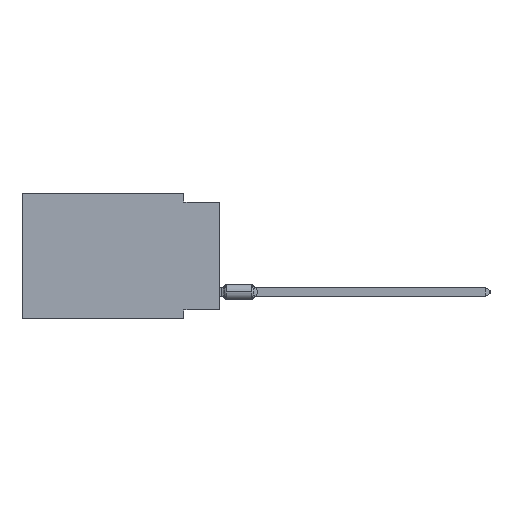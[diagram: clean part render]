
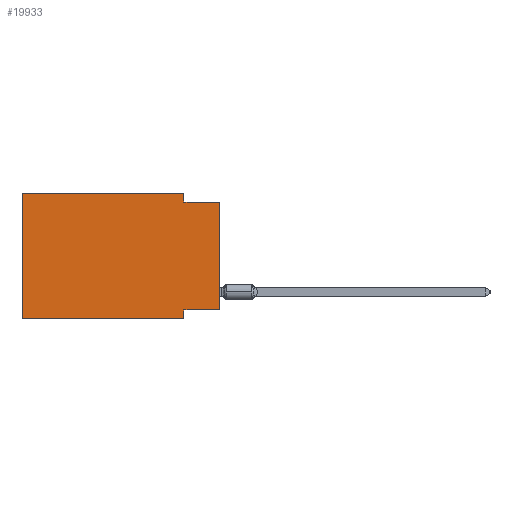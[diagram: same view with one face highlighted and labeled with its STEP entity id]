
A CAD part, left-side view. The second image highlights one B-rep face of the part: STEP entity #19933.
In plain terms, the highlighted planar face has unit normal (-1, 0, 0).
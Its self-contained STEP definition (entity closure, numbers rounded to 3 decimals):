
#3803 = DIRECTION ( 'NONE',  ( 0., 0., 1. ) ) ;
#4120 = EDGE_CURVE ( 'NONE', #29548, #60700, #34407, .T. ) ;
#5453 = VERTEX_POINT ( 'NONE', #26702 ) ;
#8085 = LINE ( 'NONE', #81244, #57320 ) ;
#9724 = CARTESIAN_POINT ( 'NONE',  ( 0., 2.54, 0. ) ) ;
#10638 = CARTESIAN_POINT ( 'NONE',  ( 0., 13.97, 0. ) ) ;
#11096 = CARTESIAN_POINT ( 'NONE',  ( 0., 2.54, -8.89 ) ) ;
#13629 = DIRECTION ( 'NONE',  ( 0., 1., 0. ) ) ;
#16205 = ORIENTED_EDGE ( 'NONE', *, *, #82289, .F. ) ;
#17096 = PLANE ( 'NONE',  #102132 ) ;
#19933 = ADVANCED_FACE ( 'NONE', ( #73169 ), #17096, .F. ) ;
#20135 = DIRECTION ( 'NONE',  ( 0., 0., -1. ) ) ;
#25701 = DIRECTION ( 'NONE',  ( 0., -1., 0. ) ) ;
#26398 = DIRECTION ( 'NONE',  ( 0., -1., 0. ) ) ;
#26702 = CARTESIAN_POINT ( 'NONE',  ( 0., 0., -8.255 ) ) ;
#27596 = VECTOR ( 'NONE', #26398, 1000. ) ;
#27738 = CARTESIAN_POINT ( 'NONE',  ( 0., 0., -0.635 ) ) ;
#28299 = ORIENTED_EDGE ( 'NONE', *, *, #104268, .T. ) ;
#28945 = EDGE_CURVE ( 'NONE', #60700, #82706, #66295, .T. ) ;
#29548 = VERTEX_POINT ( 'NONE', #10638 ) ;
#31070 = ORIENTED_EDGE ( 'NONE', *, *, #4120, .F. ) ;
#31104 = DIRECTION ( 'NONE',  ( 0., 0., 1. ) ) ;
#32250 = EDGE_CURVE ( 'NONE', #67128, #29548, #66833, .T. ) ;
#33915 = ORIENTED_EDGE ( 'NONE', *, *, #34545, .F. ) ;
#34407 = LINE ( 'NONE', #66945, #27596 ) ;
#34545 = EDGE_CURVE ( 'NONE', #82706, #63183, #56461, .T. ) ;
#39136 = LINE ( 'NONE', #72200, #97717 ) ;
#41253 = DIRECTION ( 'NONE',  ( 0., 0., -1. ) ) ;
#43645 = DIRECTION ( 'NONE',  ( 0., 0., -1. ) ) ;
#44591 = CARTESIAN_POINT ( 'NONE',  ( 0., 2.54, 0. ) ) ;
#45098 = CARTESIAN_POINT ( 'NONE',  ( 0., 2.54, -8.89 ) ) ;
#46465 = EDGE_CURVE ( 'NONE', #5453, #63183, #39136, .T. ) ;
#47699 = ORIENTED_EDGE ( 'NONE', *, *, #32250, .F. ) ;
#48477 = DIRECTION ( 'NONE',  ( 0., -1., 0. ) ) ;
#50919 = VECTOR ( 'NONE', #13629, 1000. ) ;
#54197 = CARTESIAN_POINT ( 'NONE',  ( 0., 0., -8.255 ) ) ;
#56028 = VECTOR ( 'NONE', #3803, 1000. ) ;
#56461 = LINE ( 'NONE', #89075, #79188 ) ;
#57320 = VECTOR ( 'NONE', #25701, 1000. ) ;
#59254 = CARTESIAN_POINT ( 'NONE',  ( 0., 2.54, -8.255 ) ) ;
#60700 = VERTEX_POINT ( 'NONE', #44591 ) ;
#61387 = ORIENTED_EDGE ( 'NONE', *, *, #85393, .F. ) ;
#63183 = VERTEX_POINT ( 'NONE', #27738 ) ;
#63993 = VERTEX_POINT ( 'NONE', #45098 ) ;
#64300 = VERTEX_POINT ( 'NONE', #59254 ) ;
#65143 = CARTESIAN_POINT ( 'NONE',  ( 0., 13.97, 0. ) ) ;
#65835 = CARTESIAN_POINT ( 'NONE',  ( 0., 2.54, -0.635 ) ) ;
#66295 = LINE ( 'NONE', #9724, #91425 ) ;
#66833 = LINE ( 'NONE', #76965, #56028 ) ;
#66945 = CARTESIAN_POINT ( 'NONE',  ( 0., 13.97, 0. ) ) ;
#67128 = VERTEX_POINT ( 'NONE', #101064 ) ;
#67742 = EDGE_LOOP ( 'NONE', ( #97123, #33915, #92572, #31070, #47699, #28299, #16205, #61387 ) ) ;
#72200 = CARTESIAN_POINT ( 'NONE',  ( 0., 0., 0. ) ) ;
#73169 = FACE_OUTER_BOUND ( 'NONE', #67742, .T. ) ;
#76965 = CARTESIAN_POINT ( 'NONE',  ( 0., 13.97, 0. ) ) ;
#79188 = VECTOR ( 'NONE', #48477, 1000. ) ;
#81244 = CARTESIAN_POINT ( 'NONE',  ( 0., 13.97, -8.89 ) ) ;
#82289 = EDGE_CURVE ( 'NONE', #64300, #63993, #101361, .T. ) ;
#82706 = VERTEX_POINT ( 'NONE', #65835 ) ;
#85393 = EDGE_CURVE ( 'NONE', #5453, #64300, #104452, .T. ) ;
#89075 = CARTESIAN_POINT ( 'NONE',  ( 0., 0., -0.635 ) ) ;
#91425 = VECTOR ( 'NONE', #41253, 1000. ) ;
#92572 = ORIENTED_EDGE ( 'NONE', *, *, #28945, .F. ) ;
#95017 = VECTOR ( 'NONE', #20135, 1000. ) ;
#97123 = ORIENTED_EDGE ( 'NONE', *, *, #46465, .T. ) ;
#97717 = VECTOR ( 'NONE', #31104, 1000. ) ;
#97765 = DIRECTION ( 'NONE',  ( 1., 0., 0. ) ) ;
#101064 = CARTESIAN_POINT ( 'NONE',  ( 0., 13.97, -8.89 ) ) ;
#101361 = LINE ( 'NONE', #11096, #95017 ) ;
#102132 = AXIS2_PLACEMENT_3D ( 'NONE', #65143, #97765, #43645 ) ;
#104268 = EDGE_CURVE ( 'NONE', #67128, #63993, #8085, .T. ) ;
#104452 = LINE ( 'NONE', #54197, #50919 ) ;
